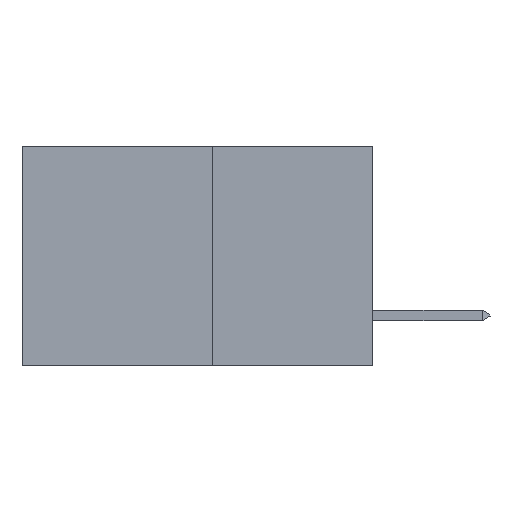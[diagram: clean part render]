
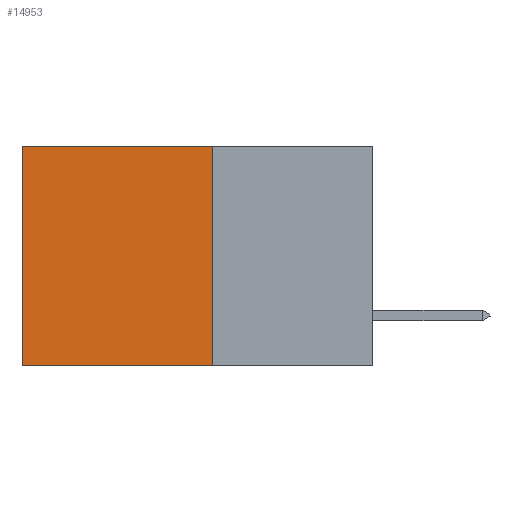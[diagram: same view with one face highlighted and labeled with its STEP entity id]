
A CAD part, left-side view. The second image highlights one B-rep face of the part: STEP entity #14953.
In plain terms, the highlighted planar face has unit normal (-1, 0, 0).
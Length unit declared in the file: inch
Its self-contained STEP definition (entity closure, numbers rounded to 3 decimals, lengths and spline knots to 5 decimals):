
#20 = DIRECTION ( 'NONE',  ( 0., 0., -1. ) ) ;
#101 = ORIENTED_EDGE ( 'NONE', *, *, #14021, .F. ) ;
#932 = VECTOR ( 'NONE', #3030, 39.37008 ) ;
#1041 = VECTOR ( 'NONE', #1175, 39.37008 ) ;
#1175 = DIRECTION ( 'NONE',  ( 0., 1., 0. ) ) ;
#1636 = CARTESIAN_POINT ( 'NONE',  ( 0.277, 0.27, -0.37 ) ) ;
#1696 = VERTEX_POINT ( 'NONE', #5221 ) ;
#2183 = ORIENTED_EDGE ( 'NONE', *, *, #13875, .F. ) ;
#2453 = DIRECTION ( 'NONE',  ( 0., 0., -1. ) ) ;
#3030 = DIRECTION ( 'NONE',  ( 0., 0., -1. ) ) ;
#5221 = CARTESIAN_POINT ( 'NONE',  ( 0.277, 0.27, 0. ) ) ;
#5538 = CARTESIAN_POINT ( 'NONE',  ( 0.277, 0.59, -0.37 ) ) ;
#6258 = VERTEX_POINT ( 'NONE', #5538 ) ;
#6721 = LINE ( 'NONE', #16416, #17190 ) ;
#7218 = LINE ( 'NONE', #16407, #10412 ) ;
#7871 = VERTEX_POINT ( 'NONE', #9134 ) ;
#8166 = DIRECTION ( 'NONE',  ( 0., 1., 0. ) ) ;
#8499 = VERTEX_POINT ( 'NONE', #10398 ) ;
#8625 = LINE ( 'NONE', #1636, #932 ) ;
#9134 = CARTESIAN_POINT ( 'NONE',  ( 0.277, 0.27, -0.37 ) ) ;
#9242 = CARTESIAN_POINT ( 'NONE',  ( 0.277, 0.27, -0.37 ) ) ;
#9253 = EDGE_CURVE ( 'NONE', #1696, #8499, #11964, .T. ) ;
#9694 = ORIENTED_EDGE ( 'NONE', *, *, #9253, .T. ) ;
#9978 = EDGE_CURVE ( 'NONE', #8499, #6258, #7218, .T. ) ;
#10082 = FACE_OUTER_BOUND ( 'NONE', #14224, .T. ) ;
#10398 = CARTESIAN_POINT ( 'NONE',  ( 0.277, 0.59, 0. ) ) ;
#10412 = VECTOR ( 'NONE', #20, 39.37008 ) ;
#10638 = DIRECTION ( 'NONE',  ( 1., 0., 0. ) ) ;
#11964 = LINE ( 'NONE', #12137, #1041 ) ;
#12137 = CARTESIAN_POINT ( 'NONE',  ( 0.277, 0.27, 0. ) ) ;
#12238 = AXIS2_PLACEMENT_3D ( 'NONE', #9242, #10638, #2453 ) ;
#13875 = EDGE_CURVE ( 'NONE', #7871, #6258, #6721, .T. ) ;
#14021 = EDGE_CURVE ( 'NONE', #1696, #7871, #8625, .T. ) ;
#14224 = EDGE_LOOP ( 'NONE', ( #15879, #2183, #101, #9694 ) ) ;
#14953 = ADVANCED_FACE ( 'NONE', ( #10082 ), #17450, .F. ) ;
#15879 = ORIENTED_EDGE ( 'NONE', *, *, #9978, .T. ) ;
#16407 = CARTESIAN_POINT ( 'NONE',  ( 0.277, 0.59, -0.37 ) ) ;
#16416 = CARTESIAN_POINT ( 'NONE',  ( 0.277, 0.27, -0.37 ) ) ;
#17190 = VECTOR ( 'NONE', #8166, 39.37008 ) ;
#17450 = PLANE ( 'NONE',  #12238 ) ;
